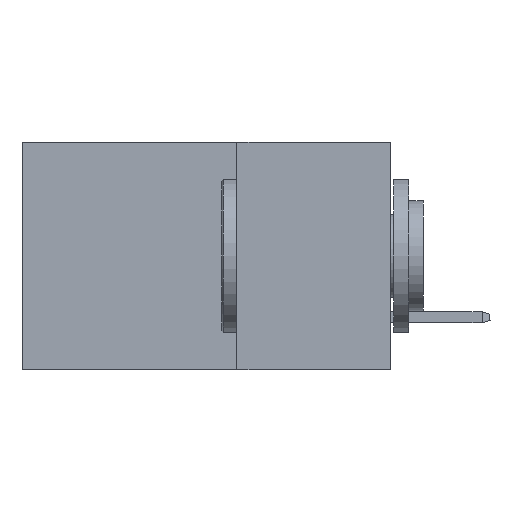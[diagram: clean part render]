
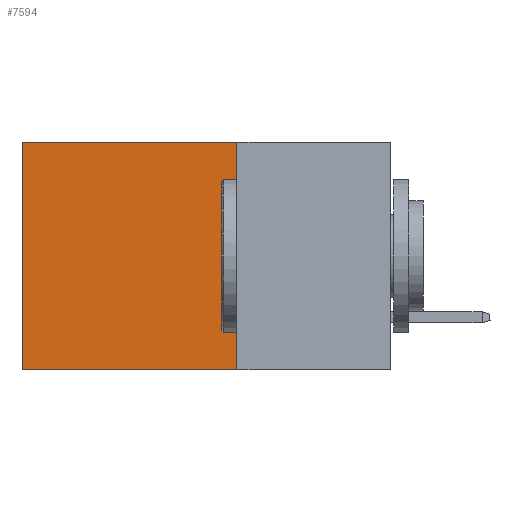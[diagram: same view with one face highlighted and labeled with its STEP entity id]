
A CAD part, left-side view. The second image highlights one B-rep face of the part: STEP entity #7594.
In plain terms, the highlighted planar face has unit normal (-1, 0, 0).
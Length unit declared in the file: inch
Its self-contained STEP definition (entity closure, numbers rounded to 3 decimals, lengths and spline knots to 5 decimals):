
#311 = ORIENTED_EDGE ( 'NONE', *, *, #6317, .T. ) ;
#474 = DIRECTION ( 'NONE',  ( 0., 0., -1. ) ) ;
#890 = CARTESIAN_POINT ( 'NONE',  ( 0.2875, 0.6, -0.37 ) ) ;
#1314 = VECTOR ( 'NONE', #1754, 39.37008 ) ;
#1367 = VECTOR ( 'NONE', #3320, 39.37008 ) ;
#1475 = LINE ( 'NONE', #10876, #13637 ) ;
#1537 = FACE_OUTER_BOUND ( 'NONE', #9778, .T. ) ;
#1581 = DIRECTION ( 'NONE',  ( 1., 0., 0. ) ) ;
#1602 = EDGE_CURVE ( 'NONE', #8944, #10400, #1475, .T. ) ;
#1754 = DIRECTION ( 'NONE',  ( 0., 1., 0. ) ) ;
#2011 = DIRECTION ( 'NONE',  ( 0., 0., -1. ) ) ;
#2693 = CARTESIAN_POINT ( 'NONE',  ( 0.2875, 0.6, 0. ) ) ;
#3320 = DIRECTION ( 'NONE',  ( 0., 1., 0. ) ) ;
#3407 = VERTEX_POINT ( 'NONE', #890 ) ;
#3575 = CARTESIAN_POINT ( 'NONE',  ( 0.2875, 0.6, 0. ) ) ;
#3798 = PLANE ( 'NONE',  #8449 ) ;
#4424 = CARTESIAN_POINT ( 'NONE',  ( 0.2875, 0.25, -0.37 ) ) ;
#4660 = LINE ( 'NONE', #4424, #1367 ) ;
#5958 = DIRECTION ( 'NONE',  ( 0., 0., -1. ) ) ;
#6317 = EDGE_CURVE ( 'NONE', #8944, #14364, #12984, .T. ) ;
#7264 = EDGE_CURVE ( 'NONE', #14364, #3407, #14255, .T. ) ;
#7594 = ADVANCED_FACE ( 'NONE', ( #1537 ), #3798, .F. ) ;
#8101 = CARTESIAN_POINT ( 'NONE',  ( 0.2875, 0.25, 0. ) ) ;
#8360 = CARTESIAN_POINT ( 'NONE',  ( 0.2875, 0.25, 0. ) ) ;
#8449 = AXIS2_PLACEMENT_3D ( 'NONE', #8360, #1581, #5958 ) ;
#8486 = CARTESIAN_POINT ( 'NONE',  ( 0.2875, 0.25, 0. ) ) ;
#8944 = VERTEX_POINT ( 'NONE', #8101 ) ;
#8966 = ORIENTED_EDGE ( 'NONE', *, *, #1602, .F. ) ;
#9778 = EDGE_LOOP ( 'NONE', ( #11512, #10897, #8966, #311 ) ) ;
#10400 = VERTEX_POINT ( 'NONE', #11337 ) ;
#10596 = VECTOR ( 'NONE', #474, 39.37008 ) ;
#10876 = CARTESIAN_POINT ( 'NONE',  ( 0.2875, 0.25, 0. ) ) ;
#10897 = ORIENTED_EDGE ( 'NONE', *, *, #12432, .F. ) ;
#11337 = CARTESIAN_POINT ( 'NONE',  ( 0.2875, 0.25, -0.37 ) ) ;
#11512 = ORIENTED_EDGE ( 'NONE', *, *, #7264, .T. ) ;
#12432 = EDGE_CURVE ( 'NONE', #10400, #3407, #4660, .T. ) ;
#12984 = LINE ( 'NONE', #8486, #1314 ) ;
#13637 = VECTOR ( 'NONE', #2011, 39.37008 ) ;
#14255 = LINE ( 'NONE', #3575, #10596 ) ;
#14364 = VERTEX_POINT ( 'NONE', #2693 ) ;
